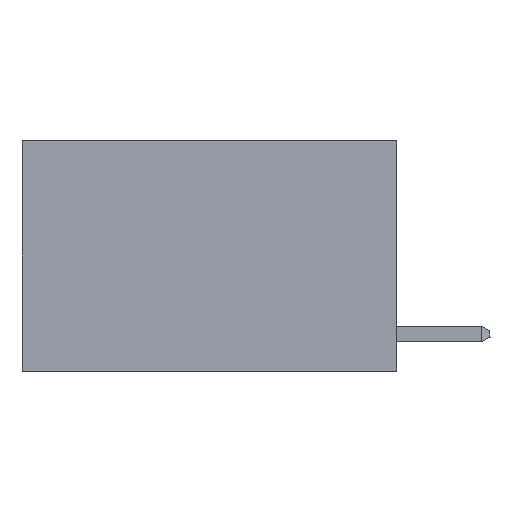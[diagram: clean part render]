
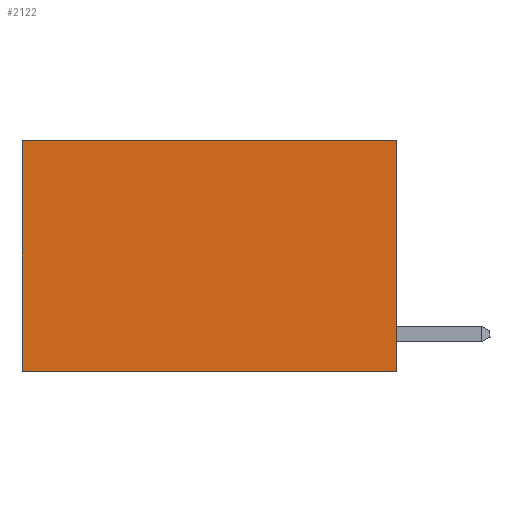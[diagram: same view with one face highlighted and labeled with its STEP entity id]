
A CAD part, left-side view. The second image highlights one B-rep face of the part: STEP entity #2122.
In plain terms, the highlighted planar face has unit normal (-1, 0, 0).
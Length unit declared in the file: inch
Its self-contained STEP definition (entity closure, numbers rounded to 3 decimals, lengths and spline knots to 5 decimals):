
#150 = CARTESIAN_POINT ( 'NONE',  ( 0.2625, 0., 0. ) ) ;
#1075 = EDGE_CURVE ( 'NONE', #11324, #6165, #27130, .T. ) ;
#1372 = ORIENTED_EDGE ( 'NONE', *, *, #7884, .T. ) ;
#2122 = ADVANCED_FACE ( 'NONE', ( #6054 ), #22198, .F. ) ;
#2330 = DIRECTION ( 'NONE',  ( 0., 0., -1. ) ) ;
#3593 = AXIS2_PLACEMENT_3D ( 'NONE', #4010, #10699, #29027 ) ;
#3633 = DIRECTION ( 'NONE',  ( 0., 0., -1. ) ) ;
#4010 = CARTESIAN_POINT ( 'NONE',  ( 0.2625, 0., 0. ) ) ;
#5325 = CARTESIAN_POINT ( 'NONE',  ( 0.2625, 0.6, -0.37 ) ) ;
#5817 = VERTEX_POINT ( 'NONE', #28397 ) ;
#5961 = LINE ( 'NONE', #16288, #20335 ) ;
#6054 = FACE_OUTER_BOUND ( 'NONE', #25883, .T. ) ;
#6165 = VERTEX_POINT ( 'NONE', #28455 ) ;
#7884 = EDGE_CURVE ( 'NONE', #11324, #5817, #29693, .T. ) ;
#8993 = VECTOR ( 'NONE', #3633, 39.37008 ) ;
#10699 = DIRECTION ( 'NONE',  ( 1., 0., 0. ) ) ;
#10773 = CARTESIAN_POINT ( 'NONE',  ( 0.2625, 0., 0. ) ) ;
#11324 = VERTEX_POINT ( 'NONE', #23108 ) ;
#14702 = LINE ( 'NONE', #24037, #8993 ) ;
#15401 = DIRECTION ( 'NONE',  ( 0., 1., 0. ) ) ;
#16288 = CARTESIAN_POINT ( 'NONE',  ( 0.2625, 0., -0.37 ) ) ;
#16443 = EDGE_CURVE ( 'NONE', #5817, #26602, #14702, .T. ) ;
#19599 = ORIENTED_EDGE ( 'NONE', *, *, #1075, .F. ) ;
#20335 = VECTOR ( 'NONE', #27980, 39.37008 ) ;
#20557 = ORIENTED_EDGE ( 'NONE', *, *, #16443, .T. ) ;
#21038 = VECTOR ( 'NONE', #2330, 39.37008 ) ;
#22198 = PLANE ( 'NONE',  #3593 ) ;
#23108 = CARTESIAN_POINT ( 'NONE',  ( 0.2625, 0., 0. ) ) ;
#23944 = EDGE_CURVE ( 'NONE', #6165, #26602, #5961, .T. ) ;
#24037 = CARTESIAN_POINT ( 'NONE',  ( 0.2625, 0.6, 0. ) ) ;
#24694 = VECTOR ( 'NONE', #15401, 39.37008 ) ;
#25883 = EDGE_LOOP ( 'NONE', ( #20557, #26695, #19599, #1372 ) ) ;
#26602 = VERTEX_POINT ( 'NONE', #5325 ) ;
#26695 = ORIENTED_EDGE ( 'NONE', *, *, #23944, .F. ) ;
#27130 = LINE ( 'NONE', #150, #21038 ) ;
#27980 = DIRECTION ( 'NONE',  ( 0., 1., 0. ) ) ;
#28397 = CARTESIAN_POINT ( 'NONE',  ( 0.2625, 0.6, 0. ) ) ;
#28455 = CARTESIAN_POINT ( 'NONE',  ( 0.2625, 0., -0.37 ) ) ;
#29027 = DIRECTION ( 'NONE',  ( 0., 0., -1. ) ) ;
#29693 = LINE ( 'NONE', #10773, #24694 ) ;
